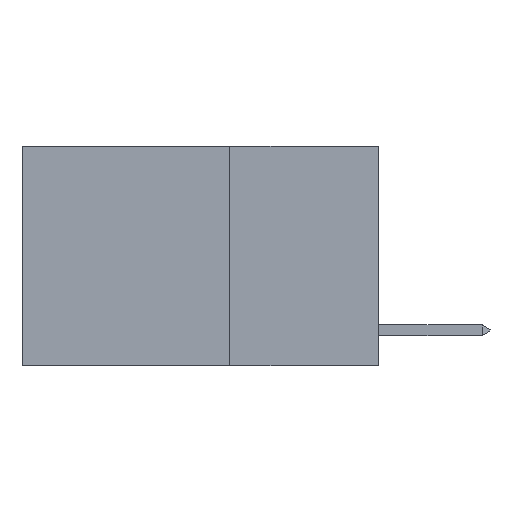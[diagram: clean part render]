
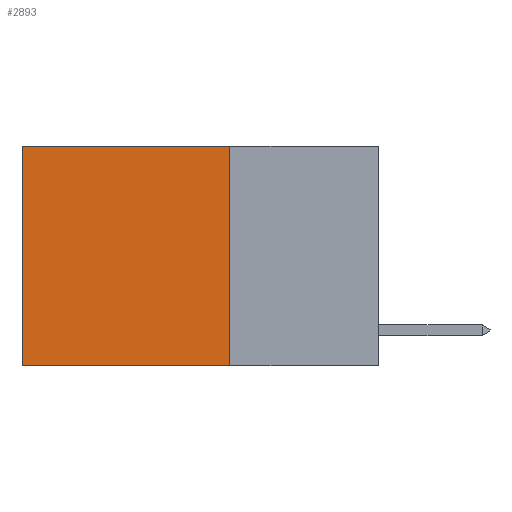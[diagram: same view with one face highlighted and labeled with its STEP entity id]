
A CAD part, left-side view. The second image highlights one B-rep face of the part: STEP entity #2893.
In plain terms, the highlighted planar face has unit normal (-1, 0, 0).
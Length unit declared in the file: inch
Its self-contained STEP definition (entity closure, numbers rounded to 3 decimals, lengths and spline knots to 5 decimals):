
#571 = LINE ( 'NONE', #9907, #10038 ) ;
#779 = FACE_OUTER_BOUND ( 'NONE', #7940, .T. ) ;
#1903 = LINE ( 'NONE', #11038, #11694 ) ;
#2468 = VECTOR ( 'NONE', #12799, 39.37008 ) ;
#2893 = ADVANCED_FACE ( 'NONE', ( #779 ), #12223, .F. ) ;
#3055 = EDGE_CURVE ( 'NONE', #9795, #3581, #14670, .T. ) ;
#3581 = VERTEX_POINT ( 'NONE', #13620 ) ;
#3690 = CARTESIAN_POINT ( 'NONE',  ( 0.2625, 0.25, -0.37 ) ) ;
#4085 = EDGE_CURVE ( 'NONE', #4506, #3581, #1903, .T. ) ;
#4506 = VERTEX_POINT ( 'NONE', #9352 ) ;
#4874 = CARTESIAN_POINT ( 'NONE',  ( 0.2625, 0.25, 0. ) ) ;
#5739 = LINE ( 'NONE', #15068, #2468 ) ;
#6117 = DIRECTION ( 'NONE',  ( 1., 0., 0. ) ) ;
#6232 = ORIENTED_EDGE ( 'NONE', *, *, #14687, .T. ) ;
#7895 = VECTOR ( 'NONE', #11310, 39.37008 ) ;
#7940 = EDGE_LOOP ( 'NONE', ( #9463, #10512, #8840, #6232 ) ) ;
#8840 = ORIENTED_EDGE ( 'NONE', *, *, #13130, .F. ) ;
#8846 = CARTESIAN_POINT ( 'NONE',  ( 0.2625, 0.25, -0.37 ) ) ;
#9352 = CARTESIAN_POINT ( 'NONE',  ( 0.2625, 0.6, 0. ) ) ;
#9463 = ORIENTED_EDGE ( 'NONE', *, *, #4085, .T. ) ;
#9795 = VERTEX_POINT ( 'NONE', #3690 ) ;
#9907 = CARTESIAN_POINT ( 'NONE',  ( 0.2625, 0.25, 0. ) ) ;
#10038 = VECTOR ( 'NONE', #14620, 39.37008 ) ;
#10512 = ORIENTED_EDGE ( 'NONE', *, *, #3055, .F. ) ;
#11038 = CARTESIAN_POINT ( 'NONE',  ( 0.2625, 0.6, 0. ) ) ;
#11310 = DIRECTION ( 'NONE',  ( 0., 1., 0. ) ) ;
#11694 = VECTOR ( 'NONE', #12246, 39.37008 ) ;
#12223 = PLANE ( 'NONE',  #12471 ) ;
#12246 = DIRECTION ( 'NONE',  ( 0., 0., -1. ) ) ;
#12410 = CARTESIAN_POINT ( 'NONE',  ( 0.2625, 0.25, 0. ) ) ;
#12471 = AXIS2_PLACEMENT_3D ( 'NONE', #4874, #6117, #14553 ) ;
#12518 = VERTEX_POINT ( 'NONE', #12410 ) ;
#12799 = DIRECTION ( 'NONE',  ( 0., 1., 0. ) ) ;
#13130 = EDGE_CURVE ( 'NONE', #12518, #9795, #571, .T. ) ;
#13620 = CARTESIAN_POINT ( 'NONE',  ( 0.2625, 0.6, -0.37 ) ) ;
#14553 = DIRECTION ( 'NONE',  ( 0., 0., -1. ) ) ;
#14620 = DIRECTION ( 'NONE',  ( 0., 0., -1. ) ) ;
#14670 = LINE ( 'NONE', #8846, #7895 ) ;
#14687 = EDGE_CURVE ( 'NONE', #12518, #4506, #5739, .T. ) ;
#15068 = CARTESIAN_POINT ( 'NONE',  ( 0.2625, 0.25, 0. ) ) ;
